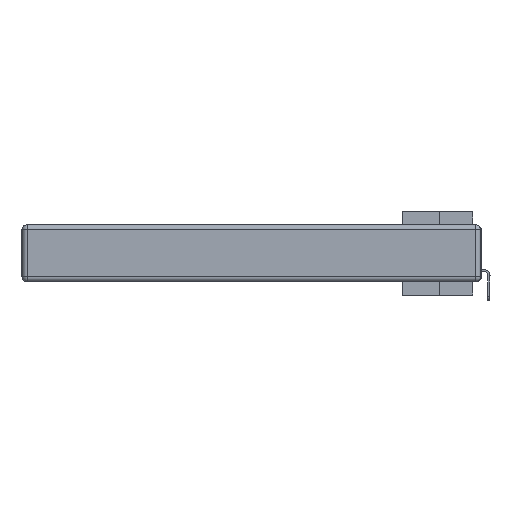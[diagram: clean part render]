
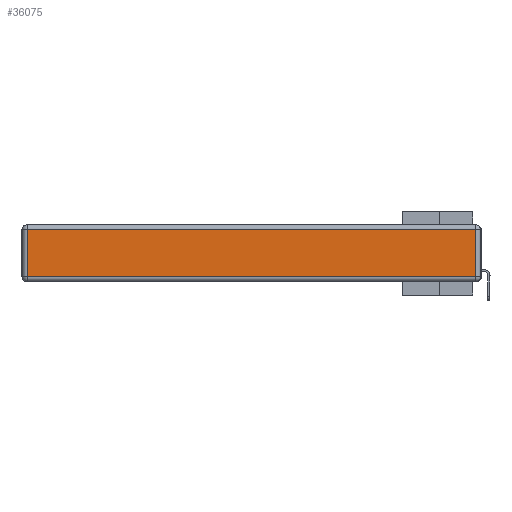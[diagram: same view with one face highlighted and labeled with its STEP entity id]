
A CAD part, left-side view. The second image highlights one B-rep face of the part: STEP entity #36075.
In plain terms, the highlighted planar face has unit normal (-1, 0, 0).
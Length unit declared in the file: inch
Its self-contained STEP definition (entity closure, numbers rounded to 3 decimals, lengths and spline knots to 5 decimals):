
#1789 = AXIS2_PLACEMENT_3D ( 'NONE', #10824, #32942, #10641 ) ;
#1877 = EDGE_CURVE ( 'NONE', #32396, #32914, #19697, .T. ) ;
#2109 = FACE_OUTER_BOUND ( 'NONE', #12744, .T. ) ;
#3573 = LINE ( 'NONE', #12458, #29958 ) ;
#4064 = CARTESIAN_POINT ( 'NONE',  ( 0., 2.72, -0.03 ) ) ;
#4558 = VERTEX_POINT ( 'NONE', #28119 ) ;
#4730 = CARTESIAN_POINT ( 'NONE',  ( 0., 0.03, -0.03 ) ) ;
#7323 = PLANE ( 'NONE',  #1789 ) ;
#9649 = ORIENTED_EDGE ( 'NONE', *, *, #15175, .T. ) ;
#10218 = EDGE_CURVE ( 'NONE', #11703, #32396, #3573, .T. ) ;
#10538 = CARTESIAN_POINT ( 'NONE',  ( 0., 0., -0.313 ) ) ;
#10641 = DIRECTION ( 'NONE',  ( 0., 0., 1. ) ) ;
#10824 = CARTESIAN_POINT ( 'NONE',  ( 0., 0., -0.343 ) ) ;
#10998 = CARTESIAN_POINT ( 'NONE',  ( 0., 2.72, -0.343 ) ) ;
#11703 = VERTEX_POINT ( 'NONE', #4730 ) ;
#11766 = VECTOR ( 'NONE', #21663, 39.37008 ) ;
#12458 = CARTESIAN_POINT ( 'NONE',  ( 0., 2.75, -0.03 ) ) ;
#12744 = EDGE_LOOP ( 'NONE', ( #16033, #9649, #24044, #13494 ) ) ;
#12967 = VECTOR ( 'NONE', #33387, 39.37008 ) ;
#13494 = ORIENTED_EDGE ( 'NONE', *, *, #1877, .T. ) ;
#15081 = EDGE_CURVE ( 'NONE', #32914, #4558, #19067, .T. ) ;
#15175 = EDGE_CURVE ( 'NONE', #4558, #11703, #36167, .T. ) ;
#16033 = ORIENTED_EDGE ( 'NONE', *, *, #15081, .T. ) ;
#19067 = LINE ( 'NONE', #10538, #12967 ) ;
#19697 = LINE ( 'NONE', #10998, #29038 ) ;
#21663 = DIRECTION ( 'NONE',  ( 0., 0., 1. ) ) ;
#22027 = CARTESIAN_POINT ( 'NONE',  ( 0., 0.03, -0.343 ) ) ;
#24044 = ORIENTED_EDGE ( 'NONE', *, *, #10218, .T. ) ;
#28119 = CARTESIAN_POINT ( 'NONE',  ( 0., 0.03, -0.313 ) ) ;
#28241 = CARTESIAN_POINT ( 'NONE',  ( 0., 2.72, -0.313 ) ) ;
#29038 = VECTOR ( 'NONE', #31235, 39.37008 ) ;
#29958 = VECTOR ( 'NONE', #32161, 39.37008 ) ;
#31235 = DIRECTION ( 'NONE',  ( 0., 0., -1. ) ) ;
#32161 = DIRECTION ( 'NONE',  ( 0., 1., 0. ) ) ;
#32396 = VERTEX_POINT ( 'NONE', #4064 ) ;
#32914 = VERTEX_POINT ( 'NONE', #28241 ) ;
#32942 = DIRECTION ( 'NONE',  ( -1., 0., 0. ) ) ;
#33387 = DIRECTION ( 'NONE',  ( 0., -1., 0. ) ) ;
#36075 = ADVANCED_FACE ( 'NONE', ( #2109 ), #7323, .T. ) ;
#36167 = LINE ( 'NONE', #22027, #11766 ) ;
